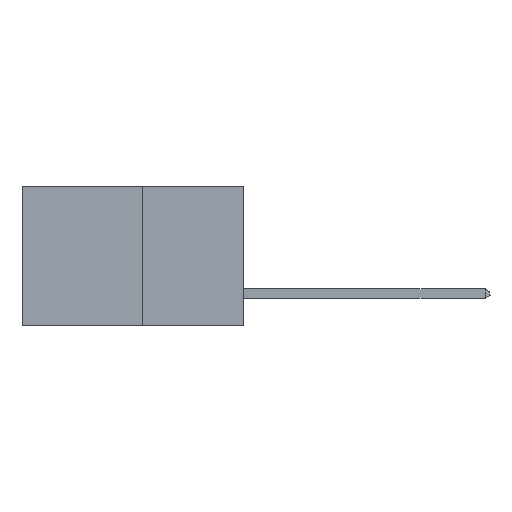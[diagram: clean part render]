
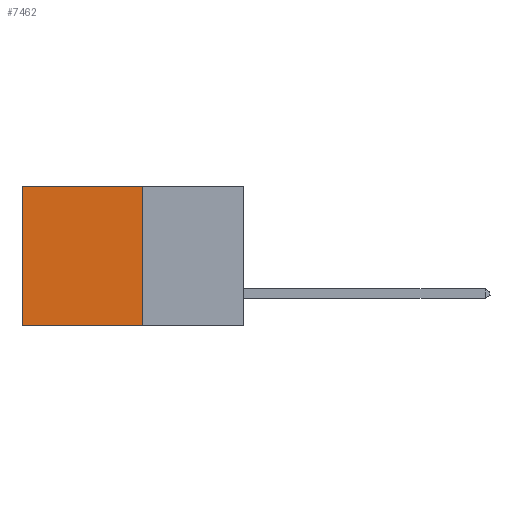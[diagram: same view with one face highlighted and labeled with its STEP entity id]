
A CAD part, left-side view. The second image highlights one B-rep face of the part: STEP entity #7462.
In plain terms, the highlighted planar face has unit normal (-1, 0, 0).
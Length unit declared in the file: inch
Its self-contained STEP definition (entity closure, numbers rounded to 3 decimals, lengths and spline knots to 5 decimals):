
#187 = ORIENTED_EDGE ( 'NONE', *, *, #8365, .F. ) ;
#749 = AXIS2_PLACEMENT_3D ( 'NONE', #10971, #10959, #10910 ) ;
#1524 = VECTOR ( 'NONE', #3210, 39.37008 ) ;
#2098 = ORIENTED_EDGE ( 'NONE', *, *, #5403, .T. ) ;
#2667 = ORIENTED_EDGE ( 'NONE', *, *, #6720, .T. ) ;
#2865 = CARTESIAN_POINT ( 'NONE',  ( 0.277, 0.27, -0.37 ) ) ;
#3210 = DIRECTION ( 'NONE',  ( 0., 1., 0. ) ) ;
#3241 = CARTESIAN_POINT ( 'NONE',  ( 0.277, 0.59, -0.37 ) ) ;
#3288 = EDGE_CURVE ( 'NONE', #6047, #4290, #9351, .T. ) ;
#3323 = DIRECTION ( 'NONE',  ( 0., 1., 0. ) ) ;
#3324 = DIRECTION ( 'NONE',  ( 0., 0., -1. ) ) ;
#3398 = CARTESIAN_POINT ( 'NONE',  ( 0.277, 0.27, 0. ) ) ;
#3568 = VERTEX_POINT ( 'NONE', #7211 ) ;
#3939 = VECTOR ( 'NONE', #7045, 39.37008 ) ;
#4085 = LINE ( 'NONE', #3241, #6134 ) ;
#4264 = FACE_OUTER_BOUND ( 'NONE', #5029, .T. ) ;
#4290 = VERTEX_POINT ( 'NONE', #5896 ) ;
#5029 = EDGE_LOOP ( 'NONE', ( #2098, #9382, #187, #2667 ) ) ;
#5403 = EDGE_CURVE ( 'NONE', #3568, #4290, #4085, .T. ) ;
#5896 = CARTESIAN_POINT ( 'NONE',  ( 0.277, 0.59, -0.37 ) ) ;
#6047 = VERTEX_POINT ( 'NONE', #8308 ) ;
#6134 = VECTOR ( 'NONE', #3324, 39.37008 ) ;
#6720 = EDGE_CURVE ( 'NONE', #9596, #3568, #8591, .T. ) ;
#7045 = DIRECTION ( 'NONE',  ( 0., 0., -1. ) ) ;
#7211 = CARTESIAN_POINT ( 'NONE',  ( 0.277, 0.59, 0. ) ) ;
#7462 = ADVANCED_FACE ( 'NONE', ( #4264 ), #11156, .F. ) ;
#8308 = CARTESIAN_POINT ( 'NONE',  ( 0.277, 0.27, -0.37 ) ) ;
#8349 = LINE ( 'NONE', #9643, #3939 ) ;
#8365 = EDGE_CURVE ( 'NONE', #9596, #6047, #8349, .T. ) ;
#8591 = LINE ( 'NONE', #3398, #1524 ) ;
#9351 = LINE ( 'NONE', #2865, #11354 ) ;
#9382 = ORIENTED_EDGE ( 'NONE', *, *, #3288, .F. ) ;
#9596 = VERTEX_POINT ( 'NONE', #10532 ) ;
#9643 = CARTESIAN_POINT ( 'NONE',  ( 0.277, 0.27, -0.37 ) ) ;
#10532 = CARTESIAN_POINT ( 'NONE',  ( 0.277, 0.27, 0. ) ) ;
#10910 = DIRECTION ( 'NONE',  ( 0., 0., -1. ) ) ;
#10959 = DIRECTION ( 'NONE',  ( 1., 0., 0. ) ) ;
#10971 = CARTESIAN_POINT ( 'NONE',  ( 0.277, 0.27, -0.37 ) ) ;
#11156 = PLANE ( 'NONE',  #749 ) ;
#11354 = VECTOR ( 'NONE', #3323, 39.37008 ) ;
